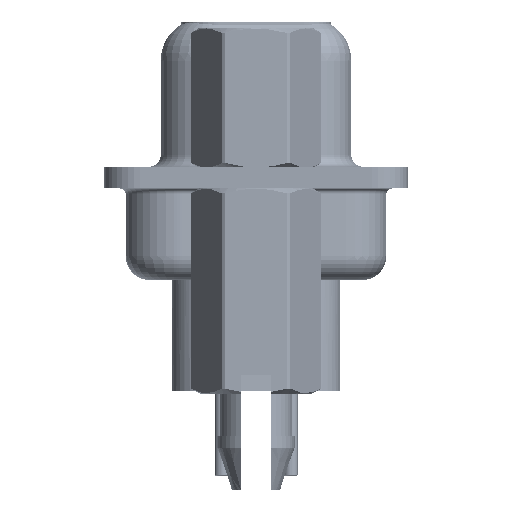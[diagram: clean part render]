
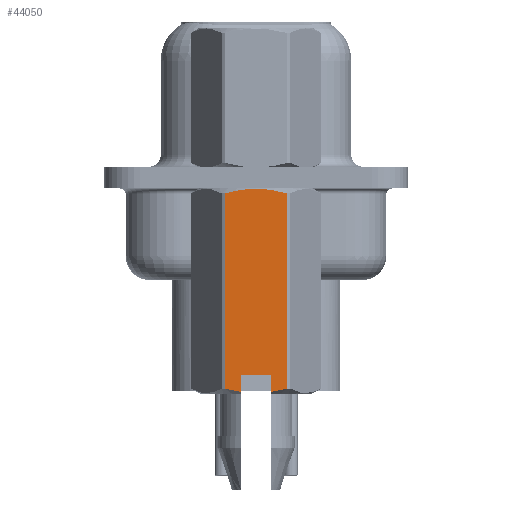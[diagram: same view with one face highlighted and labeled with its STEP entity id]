
A CAD part, left-side view. The second image highlights one B-rep face of the part: STEP entity #44050.
In plain terms, the highlighted planar face has unit normal (-1, 0, 0).
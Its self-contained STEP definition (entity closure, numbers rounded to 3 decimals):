
#79 = LINE ( 'NONE', #49477, #33444 ) ;
#639 = CARTESIAN_POINT ( 'NONE',  ( -2.381, -1.273, -0.652 ) ) ;
#2619 = VERTEX_POINT ( 'NONE', #42293 ) ;
#3340 = EDGE_CURVE ( 'NONE', #49259, #14517, #9904, .T. ) ;
#5547 = CARTESIAN_POINT ( 'NONE',  ( -2.381, -0.625, -8.2 ) ) ;
#6514 = CARTESIAN_POINT ( 'NONE',  ( -2.381, -1.06, -8.806 ) ) ;
#6574 = CARTESIAN_POINT ( 'NONE',  ( -2.381, 0., -0.468 ) ) ;
#6847 = CARTESIAN_POINT ( 'NONE',  ( -2.381, -0.215, -0.468 ) ) ;
#7952 = AXIS2_PLACEMENT_3D ( 'NONE', #28289, #11624, #11901 ) ;
#8479 = VERTEX_POINT ( 'NONE', #39285 ) ;
#8775 = VERTEX_POINT ( 'NONE', #41429 ) ;
#9061 = VERTEX_POINT ( 'NONE', #26437 ) ;
#9580 = CARTESIAN_POINT ( 'NONE',  ( -2.381, 0.845, -8.853 ) ) ;
#9904 = LINE ( 'NONE', #5547, #27787 ) ;
#11413 = EDGE_CURVE ( 'NONE', #49259, #30251, #30739, .T. ) ;
#11452 = CARTESIAN_POINT ( 'NONE',  ( -2.381, -0.625, -8.885 ) ) ;
#11624 = DIRECTION ( 'NONE',  ( -1., 0., 0. ) ) ;
#11901 = DIRECTION ( 'NONE',  ( 0., 0., 1. ) ) ;
#13232 = ORIENTED_EDGE ( 'NONE', *, *, #22515, .T. ) ;
#13375 = VERTEX_POINT ( 'NONE', #639 ) ;
#14487 = ORIENTED_EDGE ( 'NONE', *, *, #3340, .T. ) ;
#14517 = VERTEX_POINT ( 'NONE', #11452 ) ;
#16096 = ORIENTED_EDGE ( 'NONE', *, *, #36420, .T. ) ;
#16135 = CARTESIAN_POINT ( 'NONE',  ( -2.381, 0., -0.468 ) ) ;
#16409 = CARTESIAN_POINT ( 'NONE',  ( -2.381, 1.273, -0.652 ) ) ;
#17115 = EDGE_CURVE ( 'NONE', #8775, #27919, #51179, .T. ) ;
#17444 = EDGE_CURVE ( 'NONE', #8479, #9061, #23836, .T. ) ;
#18328 = VECTOR ( 'NONE', #43255, 1000. ) ;
#18699 = LINE ( 'NONE', #31773, #44869 ) ;
#19426 = CARTESIAN_POINT ( 'NONE',  ( -2.381, -0.428, -0.485 ) ) ;
#19786 = DIRECTION ( 'NONE',  ( 0., 0., -1. ) ) ;
#20709 = ORIENTED_EDGE ( 'NONE', *, *, #23278, .F. ) ;
#21573 = ORIENTED_EDGE ( 'NONE', *, *, #17115, .T. ) ;
#22327 = CARTESIAN_POINT ( 'NONE',  ( -2.381, -0.625, -8.2 ) ) ;
#22515 = EDGE_CURVE ( 'NONE', #9061, #8775, #79, .T. ) ;
#23278 = EDGE_CURVE ( 'NONE', #30251, #27919, #18699, .T. ) ;
#23836 = B_SPLINE_CURVE_WITH_KNOTS ( 'NONE', 3,
 ( #16135, #45555, #25109, #24846, #24314, #16409 ),
 .UNSPECIFIED., .F., .F.,
 ( 4, 2, 4 ),
 ( 0.004, 0.004, 0.005 ),
 .UNSPECIFIED. ) ;
#24314 = CARTESIAN_POINT ( 'NONE',  ( -2.381, 1.066, -0.596 ) ) ;
#24846 = CARTESIAN_POINT ( 'NONE',  ( -2.381, 0.858, -0.55 ) ) ;
#25109 = CARTESIAN_POINT ( 'NONE',  ( -2.381, 0.432, -0.485 ) ) ;
#25371 = CARTESIAN_POINT ( 'NONE',  ( -2.381, 0.625, -8.885 ) ) ;
#25983 = CARTESIAN_POINT ( 'NONE',  ( -2.381, 1.273, -8.748 ) ) ;
#26437 = CARTESIAN_POINT ( 'NONE',  ( -2.381, 1.273, -0.652 ) ) ;
#26591 = DIRECTION ( 'NONE',  ( 0., 0., -1. ) ) ;
#27290 = CARTESIAN_POINT ( 'NONE',  ( -2.381, -0.625, -8.885 ) ) ;
#27787 = VECTOR ( 'NONE', #26591, 1000. ) ;
#27919 = VERTEX_POINT ( 'NONE', #25371 ) ;
#28289 = CARTESIAN_POINT ( 'NONE',  ( -2.381, -1.375, 7.399 ) ) ;
#28848 = ORIENTED_EDGE ( 'NONE', *, *, #11413, .F. ) ;
#29189 = B_SPLINE_CURVE_WITH_KNOTS ( 'NONE', 3,
 ( #27290, #34903, #6514, #39795 ),
 .UNSPECIFIED., .F., .F.,
 ( 4, 4 ),
 ( 0.003, 0.004 ),
 .UNSPECIFIED. ) ;
#30251 = VERTEX_POINT ( 'NONE', #39047 ) ;
#30739 = LINE ( 'NONE', #34262, #18328 ) ;
#31161 = CARTESIAN_POINT ( 'NONE',  ( -2.381, -1.065, -0.596 ) ) ;
#31773 = CARTESIAN_POINT ( 'NONE',  ( -2.381, 0.625, -8.2 ) ) ;
#32113 = EDGE_CURVE ( 'NONE', #2619, #13375, #48031, .T. ) ;
#33444 = VECTOR ( 'NONE', #45379, 1000. ) ;
#34262 = CARTESIAN_POINT ( 'NONE',  ( -2.381, -0.625, -8.2 ) ) ;
#34903 = CARTESIAN_POINT ( 'NONE',  ( -2.381, -0.842, -8.854 ) ) ;
#36420 = EDGE_CURVE ( 'NONE', #14517, #2619, #29189, .T. ) ;
#38454 = ORIENTED_EDGE ( 'NONE', *, *, #32113, .T. ) ;
#38493 = CARTESIAN_POINT ( 'NONE',  ( -2.381, 0.625, -8.885 ) ) ;
#39047 = CARTESIAN_POINT ( 'NONE',  ( -2.381, 0.625, -8.2 ) ) ;
#39285 = CARTESIAN_POINT ( 'NONE',  ( -2.381, 0., -0.468 ) ) ;
#39795 = CARTESIAN_POINT ( 'NONE',  ( -2.381, -1.273, -8.748 ) ) ;
#40100 = CARTESIAN_POINT ( 'NONE',  ( -2.381, -1.273, 0.581 ) ) ;
#40385 = CARTESIAN_POINT ( 'NONE',  ( -2.381, -0.853, -0.549 ) ) ;
#41429 = CARTESIAN_POINT ( 'NONE',  ( -2.381, 1.273, -8.748 ) ) ;
#41450 = VECTOR ( 'NONE', #48571, 1000. ) ;
#42293 = CARTESIAN_POINT ( 'NONE',  ( -2.381, -1.273, -8.748 ) ) ;
#43255 = DIRECTION ( 'NONE',  ( 0., 1., 0. ) ) ;
#43942 = CARTESIAN_POINT ( 'NONE',  ( -2.381, -1.273, -0.652 ) ) ;
#44050 = ADVANCED_FACE ( 'NONE', ( #47933 ), #45178, .T. ) ;
#44365 = ORIENTED_EDGE ( 'NONE', *, *, #17444, .T. ) ;
#44869 = VECTOR ( 'NONE', #19786, 1000. ) ;
#45178 = PLANE ( 'NONE',  #7952 ) ;
#45379 = DIRECTION ( 'NONE',  ( 0., 0., -1. ) ) ;
#45555 = CARTESIAN_POINT ( 'NONE',  ( -2.381, 0.215, -0.468 ) ) ;
#46476 = B_SPLINE_CURVE_WITH_KNOTS ( 'NONE', 3,
 ( #43942, #31161, #40385, #19426, #6847, #6574 ),
 .UNSPECIFIED., .F., .F.,
 ( 4, 2, 4 ),
 ( 0.003, 0.003, 0.004 ),
 .UNSPECIFIED. ) ;
#47933 = FACE_OUTER_BOUND ( 'NONE', #51472, .T. ) ;
#48031 = LINE ( 'NONE', #40100, #41450 ) ;
#48571 = DIRECTION ( 'NONE',  ( 0., 0., 1. ) ) ;
#49073 = ORIENTED_EDGE ( 'NONE', *, *, #51787, .T. ) ;
#49259 = VERTEX_POINT ( 'NONE', #22327 ) ;
#49477 = CARTESIAN_POINT ( 'NONE',  ( -2.381, 1.273, 0.581 ) ) ;
#50526 = CARTESIAN_POINT ( 'NONE',  ( -2.381, 1.06, -8.806 ) ) ;
#51179 = B_SPLINE_CURVE_WITH_KNOTS ( 'NONE', 3,
 ( #25983, #50526, #9580, #38493 ),
 .UNSPECIFIED., .F., .F.,
 ( 4, 4 ),
 ( 0.001, 0.002 ),
 .UNSPECIFIED. ) ;
#51472 = EDGE_LOOP ( 'NONE', ( #20709, #28848, #14487, #16096, #38454, #49073, #44365, #13232, #21573 ) ) ;
#51787 = EDGE_CURVE ( 'NONE', #13375, #8479, #46476, .T. ) ;
